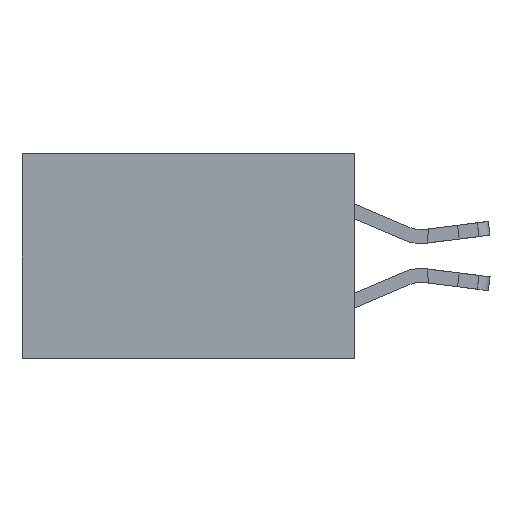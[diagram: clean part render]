
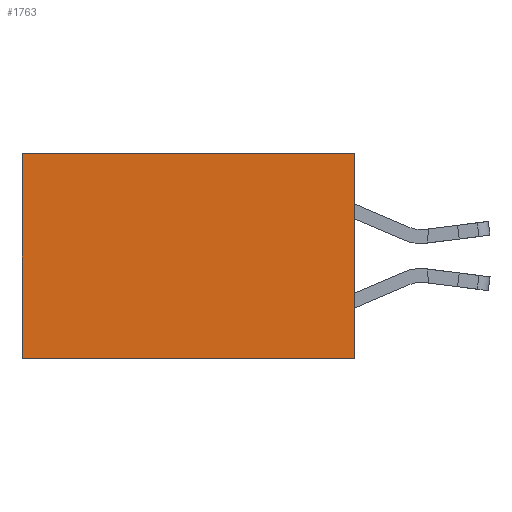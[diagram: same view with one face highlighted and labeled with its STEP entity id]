
A CAD part, left-side view. The second image highlights one B-rep face of the part: STEP entity #1763.
In plain terms, the highlighted planar face has unit normal (-1, 0, 0).
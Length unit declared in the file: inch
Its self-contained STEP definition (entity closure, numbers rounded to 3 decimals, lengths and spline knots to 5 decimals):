
#567 = CARTESIAN_POINT ( 'NONE',  ( 0.2615, 0., -0.37 ) ) ;
#1240 = EDGE_CURVE ( 'NONE', #17243, #19418, #17151, .T. ) ;
#1763 = ADVANCED_FACE ( 'NONE', ( #19353 ), #5332, .F. ) ;
#1784 = DIRECTION ( 'NONE',  ( 0., 1., 0. ) ) ;
#1788 = VECTOR ( 'NONE', #1784, 39.37008 ) ;
#2017 = ORIENTED_EDGE ( 'NONE', *, *, #9708, .T. ) ;
#2090 = AXIS2_PLACEMENT_3D ( 'NONE', #6699, #7794, #7722 ) ;
#2721 = DIRECTION ( 'NONE',  ( 0., 0., -1. ) ) ;
#2969 = CARTESIAN_POINT ( 'NONE',  ( 0.2615, 0.6, -0.37 ) ) ;
#4169 = CARTESIAN_POINT ( 'NONE',  ( 0.2615, 0., 0. ) ) ;
#4184 = VECTOR ( 'NONE', #10539, 39.37008 ) ;
#4383 = EDGE_CURVE ( 'NONE', #17243, #9191, #17527, .T. ) ;
#4756 = DIRECTION ( 'NONE',  ( 0., 0., -1. ) ) ;
#5332 = PLANE ( 'NONE',  #2090 ) ;
#5496 = CARTESIAN_POINT ( 'NONE',  ( 0.2615, 0.6, -0.37 ) ) ;
#5812 = EDGE_LOOP ( 'NONE', ( #2017, #10325, #14819, #10620 ) ) ;
#6699 = CARTESIAN_POINT ( 'NONE',  ( 0.2615, 0., -0.37 ) ) ;
#7722 = DIRECTION ( 'NONE',  ( 0., 0., -1. ) ) ;
#7794 = DIRECTION ( 'NONE',  ( 1., 0., 0. ) ) ;
#8168 = VECTOR ( 'NONE', #4756, 39.37008 ) ;
#9191 = VERTEX_POINT ( 'NONE', #10543 ) ;
#9708 = EDGE_CURVE ( 'NONE', #9191, #13777, #18094, .T. ) ;
#10325 = ORIENTED_EDGE ( 'NONE', *, *, #12581, .F. ) ;
#10539 = DIRECTION ( 'NONE',  ( 0., 1., 0. ) ) ;
#10543 = CARTESIAN_POINT ( 'NONE',  ( 0.2615, 0.6, 0. ) ) ;
#10569 = CARTESIAN_POINT ( 'NONE',  ( 0.2615, 0., 0. ) ) ;
#10620 = ORIENTED_EDGE ( 'NONE', *, *, #4383, .T. ) ;
#11324 = CARTESIAN_POINT ( 'NONE',  ( 0.2615, 0., -0.37 ) ) ;
#11631 = CARTESIAN_POINT ( 'NONE',  ( 0.2615, 0., -0.37 ) ) ;
#12581 = EDGE_CURVE ( 'NONE', #19418, #13777, #14320, .T. ) ;
#13777 = VERTEX_POINT ( 'NONE', #5496 ) ;
#13900 = VECTOR ( 'NONE', #2721, 39.37008 ) ;
#14320 = LINE ( 'NONE', #11631, #1788 ) ;
#14819 = ORIENTED_EDGE ( 'NONE', *, *, #1240, .F. ) ;
#17151 = LINE ( 'NONE', #567, #8168 ) ;
#17243 = VERTEX_POINT ( 'NONE', #4169 ) ;
#17527 = LINE ( 'NONE', #10569, #4184 ) ;
#18094 = LINE ( 'NONE', #2969, #13900 ) ;
#19353 = FACE_OUTER_BOUND ( 'NONE', #5812, .T. ) ;
#19418 = VERTEX_POINT ( 'NONE', #11324 ) ;
